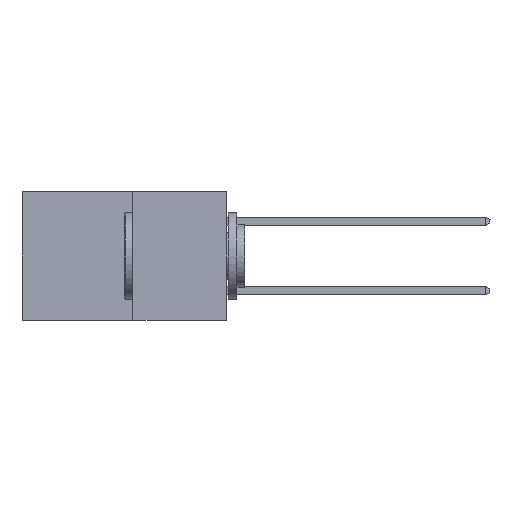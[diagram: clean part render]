
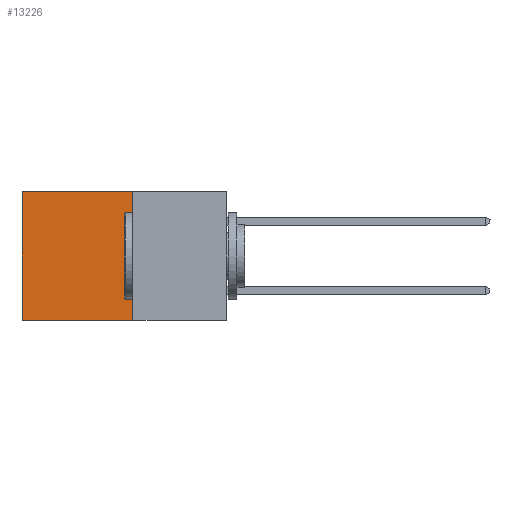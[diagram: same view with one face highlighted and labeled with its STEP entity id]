
A CAD part, left-side view. The second image highlights one B-rep face of the part: STEP entity #13226.
In plain terms, the highlighted planar face has unit normal (-1, 0, 0).
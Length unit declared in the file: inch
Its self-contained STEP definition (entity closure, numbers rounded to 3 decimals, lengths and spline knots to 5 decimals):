
#421 = CARTESIAN_POINT ( 'NONE',  ( 0.277, 0.59, 0. ) ) ;
#851 = VERTEX_POINT ( 'NONE', #2380 ) ;
#1529 = ORIENTED_EDGE ( 'NONE', *, *, #7163, .F. ) ;
#1567 = VECTOR ( 'NONE', #12105, 39.37008 ) ;
#2380 = CARTESIAN_POINT ( 'NONE',  ( 0.277, 0.27, -0.37 ) ) ;
#2510 = LINE ( 'NONE', #5228, #15355 ) ;
#2689 = DIRECTION ( 'NONE',  ( 0., 1., 0. ) ) ;
#2825 = VECTOR ( 'NONE', #2689, 39.37008 ) ;
#4553 = ORIENTED_EDGE ( 'NONE', *, *, #5511, .T. ) ;
#5223 = CARTESIAN_POINT ( 'NONE',  ( 0.277, 0.27, 0. ) ) ;
#5228 = CARTESIAN_POINT ( 'NONE',  ( 0.277, 0.59, -0.37 ) ) ;
#5399 = DIRECTION ( 'NONE',  ( 0., 0., -1. ) ) ;
#5442 = VERTEX_POINT ( 'NONE', #6380 ) ;
#5511 = EDGE_CURVE ( 'NONE', #9198, #9212, #2510, .T. ) ;
#5709 = DIRECTION ( 'NONE',  ( 0., 0., -1. ) ) ;
#6380 = CARTESIAN_POINT ( 'NONE',  ( 0.277, 0.27, 0. ) ) ;
#7163 = EDGE_CURVE ( 'NONE', #851, #9212, #8184, .T. ) ;
#8034 = FACE_OUTER_BOUND ( 'NONE', #12086, .T. ) ;
#8184 = LINE ( 'NONE', #10884, #1567 ) ;
#8508 = VECTOR ( 'NONE', #9882, 39.37008 ) ;
#8877 = EDGE_CURVE ( 'NONE', #5442, #851, #14866, .T. ) ;
#9198 = VERTEX_POINT ( 'NONE', #421 ) ;
#9212 = VERTEX_POINT ( 'NONE', #10343 ) ;
#9882 = DIRECTION ( 'NONE',  ( 0., 0., -1. ) ) ;
#10206 = PLANE ( 'NONE',  #15086 ) ;
#10343 = CARTESIAN_POINT ( 'NONE',  ( 0.277, 0.59, -0.37 ) ) ;
#10884 = CARTESIAN_POINT ( 'NONE',  ( 0.277, 0.27, -0.37 ) ) ;
#11449 = CARTESIAN_POINT ( 'NONE',  ( 0.277, 0.27, -0.37 ) ) ;
#12041 = ORIENTED_EDGE ( 'NONE', *, *, #8877, .F. ) ;
#12086 = EDGE_LOOP ( 'NONE', ( #4553, #1529, #12041, #15222 ) ) ;
#12105 = DIRECTION ( 'NONE',  ( 0., 1., 0. ) ) ;
#12639 = DIRECTION ( 'NONE',  ( 1., 0., 0. ) ) ;
#13226 = ADVANCED_FACE ( 'NONE', ( #8034 ), #10206, .F. ) ;
#13914 = EDGE_CURVE ( 'NONE', #5442, #9198, #15280, .T. ) ;
#14866 = LINE ( 'NONE', #15736, #8508 ) ;
#15086 = AXIS2_PLACEMENT_3D ( 'NONE', #11449, #12639, #5399 ) ;
#15222 = ORIENTED_EDGE ( 'NONE', *, *, #13914, .T. ) ;
#15280 = LINE ( 'NONE', #5223, #2825 ) ;
#15355 = VECTOR ( 'NONE', #5709, 39.37008 ) ;
#15736 = CARTESIAN_POINT ( 'NONE',  ( 0.277, 0.27, -0.37 ) ) ;
